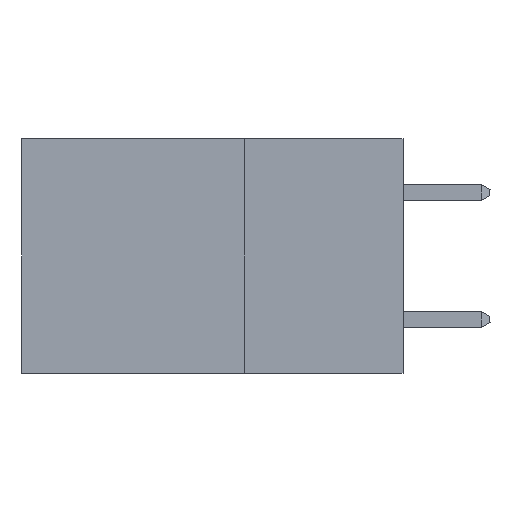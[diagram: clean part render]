
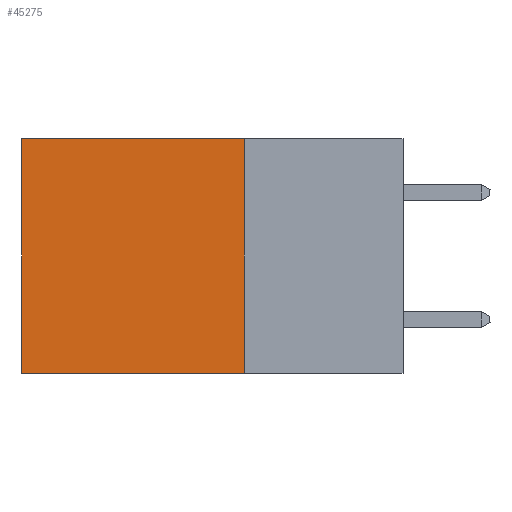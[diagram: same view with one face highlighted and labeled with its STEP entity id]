
A CAD part, left-side view. The second image highlights one B-rep face of the part: STEP entity #45275.
In plain terms, the highlighted planar face has unit normal (-1, 0, 0).
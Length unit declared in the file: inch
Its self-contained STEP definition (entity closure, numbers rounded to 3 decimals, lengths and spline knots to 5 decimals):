
#1552 = LINE ( 'NONE', #9696, #12088 ) ;
#4195 = EDGE_CURVE ( 'NONE', #9278, #40697, #20185, .T. ) ;
#9278 = VERTEX_POINT ( 'NONE', #13691 ) ;
#9696 = CARTESIAN_POINT ( 'NONE',  ( 0.2875, 0.25, 0. ) ) ;
#9918 = CARTESIAN_POINT ( 'NONE',  ( 0.2875, 0.25, -0.37 ) ) ;
#12088 = VECTOR ( 'NONE', #37325, 39.37008 ) ;
#12888 = CARTESIAN_POINT ( 'NONE',  ( 0.2875, 0.6, 0. ) ) ;
#13691 = CARTESIAN_POINT ( 'NONE',  ( 0.2875, 0.25, -0.37 ) ) ;
#14324 = FACE_OUTER_BOUND ( 'NONE', #24836, .T. ) ;
#14675 = LINE ( 'NONE', #44462, #22715 ) ;
#15874 = VECTOR ( 'NONE', #46406, 39.37008 ) ;
#16141 = VERTEX_POINT ( 'NONE', #26633 ) ;
#17943 = EDGE_CURVE ( 'NONE', #16141, #9278, #1552, .T. ) ;
#19665 = ORIENTED_EDGE ( 'NONE', *, *, #31025, .T. ) ;
#20185 = LINE ( 'NONE', #9918, #15874 ) ;
#20756 = DIRECTION ( 'NONE',  ( 0., 1., 0. ) ) ;
#22715 = VECTOR ( 'NONE', #20756, 39.37008 ) ;
#23975 = DIRECTION ( 'NONE',  ( 0., 0., -1. ) ) ;
#24836 = EDGE_LOOP ( 'NONE', ( #19665, #49382, #35165, #27428 ) ) ;
#26633 = CARTESIAN_POINT ( 'NONE',  ( 0.2875, 0.25, 0. ) ) ;
#27428 = ORIENTED_EDGE ( 'NONE', *, *, #30557, .T. ) ;
#28098 = CARTESIAN_POINT ( 'NONE',  ( 0.2875, 0.25, 0. ) ) ;
#28759 = LINE ( 'NONE', #12888, #39863 ) ;
#30557 = EDGE_CURVE ( 'NONE', #16141, #44306, #14675, .T. ) ;
#31025 = EDGE_CURVE ( 'NONE', #44306, #40697, #28759, .T. ) ;
#33881 = AXIS2_PLACEMENT_3D ( 'NONE', #28098, #36030, #23975 ) ;
#35165 = ORIENTED_EDGE ( 'NONE', *, *, #17943, .F. ) ;
#36030 = DIRECTION ( 'NONE',  ( 1., 0., 0. ) ) ;
#36365 = DIRECTION ( 'NONE',  ( 0., 0., -1. ) ) ;
#36482 = CARTESIAN_POINT ( 'NONE',  ( 0.2875, 0.6, -0.37 ) ) ;
#37325 = DIRECTION ( 'NONE',  ( 0., 0., -1. ) ) ;
#37845 = CARTESIAN_POINT ( 'NONE',  ( 0.2875, 0.6, 0. ) ) ;
#39863 = VECTOR ( 'NONE', #36365, 39.37008 ) ;
#40697 = VERTEX_POINT ( 'NONE', #36482 ) ;
#44024 = PLANE ( 'NONE',  #33881 ) ;
#44306 = VERTEX_POINT ( 'NONE', #37845 ) ;
#44462 = CARTESIAN_POINT ( 'NONE',  ( 0.2875, 0.25, 0. ) ) ;
#45275 = ADVANCED_FACE ( 'NONE', ( #14324 ), #44024, .F. ) ;
#46406 = DIRECTION ( 'NONE',  ( 0., 1., 0. ) ) ;
#49382 = ORIENTED_EDGE ( 'NONE', *, *, #4195, .F. ) ;
